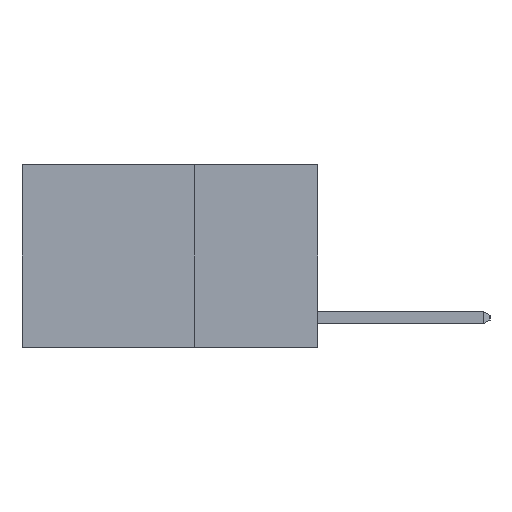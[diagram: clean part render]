
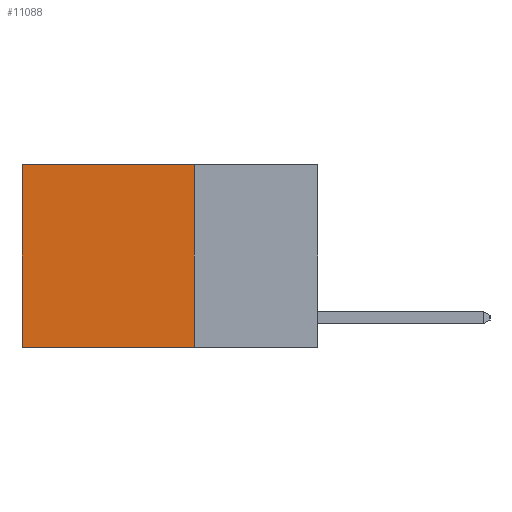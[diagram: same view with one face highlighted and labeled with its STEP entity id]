
A CAD part, left-side view. The second image highlights one B-rep face of the part: STEP entity #11088.
In plain terms, the highlighted planar face has unit normal (-1, 0, 0).
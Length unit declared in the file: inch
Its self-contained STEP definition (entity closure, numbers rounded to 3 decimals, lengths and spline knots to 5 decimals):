
#368 = DIRECTION ( 'NONE',  ( 1., 0., 0. ) ) ;
#398 = FACE_OUTER_BOUND ( 'NONE', #5554, .T. ) ;
#767 = VECTOR ( 'NONE', #10296, 39.37008 ) ;
#865 = VECTOR ( 'NONE', #2117, 39.37008 ) ;
#1179 = CARTESIAN_POINT ( 'NONE',  ( 0.2625, 0.25, -0.37 ) ) ;
#1484 = CARTESIAN_POINT ( 'NONE',  ( 0.2625, 0.25, 0. ) ) ;
#1539 = DIRECTION ( 'NONE',  ( 0., 1., 0. ) ) ;
#2117 = DIRECTION ( 'NONE',  ( 0., 0., -1. ) ) ;
#2308 = CARTESIAN_POINT ( 'NONE',  ( 0.2625, 0.6, 0. ) ) ;
#3119 = CARTESIAN_POINT ( 'NONE',  ( 0.2625, 0.25, 0. ) ) ;
#3762 = VERTEX_POINT ( 'NONE', #1179 ) ;
#3805 = EDGE_CURVE ( 'NONE', #11280, #9931, #5807, .T. ) ;
#4648 = AXIS2_PLACEMENT_3D ( 'NONE', #3119, #368, #6634 ) ;
#4872 = EDGE_CURVE ( 'NONE', #9931, #9385, #10274, .T. ) ;
#5167 = ORIENTED_EDGE ( 'NONE', *, *, #7023, .F. ) ;
#5554 = EDGE_LOOP ( 'NONE', ( #6221, #6157, #5167, #5776 ) ) ;
#5583 = LINE ( 'NONE', #5949, #767 ) ;
#5776 = ORIENTED_EDGE ( 'NONE', *, *, #3805, .T. ) ;
#5777 = PLANE ( 'NONE',  #4648 ) ;
#5807 = LINE ( 'NONE', #1484, #7547 ) ;
#5949 = CARTESIAN_POINT ( 'NONE',  ( 0.2625, 0.25, -0.37 ) ) ;
#6066 = CARTESIAN_POINT ( 'NONE',  ( 0.2625, 0.25, 0. ) ) ;
#6157 = ORIENTED_EDGE ( 'NONE', *, *, #6886, .F. ) ;
#6221 = ORIENTED_EDGE ( 'NONE', *, *, #4872, .T. ) ;
#6634 = DIRECTION ( 'NONE',  ( 0., 0., -1. ) ) ;
#6886 = EDGE_CURVE ( 'NONE', #3762, #9385, #5583, .T. ) ;
#7023 = EDGE_CURVE ( 'NONE', #11280, #3762, #10916, .T. ) ;
#7547 = VECTOR ( 'NONE', #1539, 39.37008 ) ;
#7810 = CARTESIAN_POINT ( 'NONE',  ( 0.2625, 0.6, 0. ) ) ;
#7848 = DIRECTION ( 'NONE',  ( 0., 0., -1. ) ) ;
#8522 = VECTOR ( 'NONE', #7848, 39.37008 ) ;
#9385 = VERTEX_POINT ( 'NONE', #10683 ) ;
#9931 = VERTEX_POINT ( 'NONE', #7810 ) ;
#10274 = LINE ( 'NONE', #2308, #865 ) ;
#10296 = DIRECTION ( 'NONE',  ( 0., 1., 0. ) ) ;
#10464 = CARTESIAN_POINT ( 'NONE',  ( 0.2625, 0.25, 0. ) ) ;
#10683 = CARTESIAN_POINT ( 'NONE',  ( 0.2625, 0.6, -0.37 ) ) ;
#10916 = LINE ( 'NONE', #10464, #8522 ) ;
#11088 = ADVANCED_FACE ( 'NONE', ( #398 ), #5777, .F. ) ;
#11280 = VERTEX_POINT ( 'NONE', #6066 ) ;
